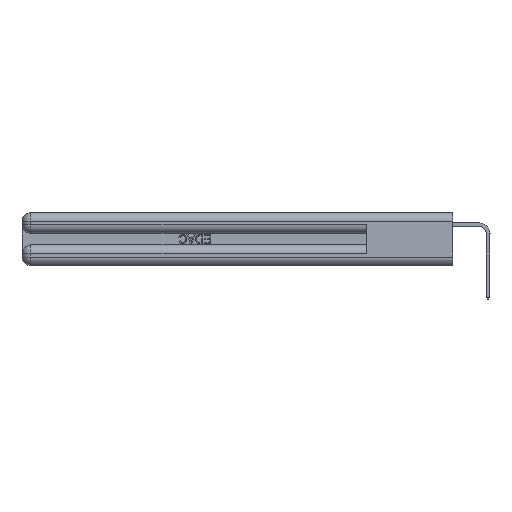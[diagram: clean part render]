
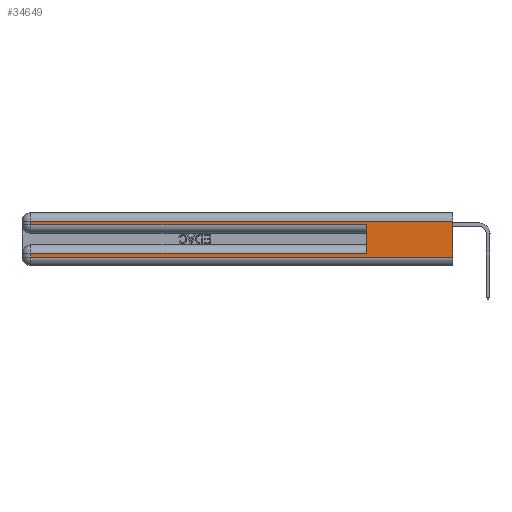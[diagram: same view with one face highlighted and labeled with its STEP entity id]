
A CAD part, left-side view. The second image highlights one B-rep face of the part: STEP entity #34649.
In plain terms, the highlighted planar face has unit normal (-1, 0, 0).
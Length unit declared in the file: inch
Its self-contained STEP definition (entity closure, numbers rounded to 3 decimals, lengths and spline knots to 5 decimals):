
#411 = CARTESIAN_POINT ( 'NONE',  ( 0., 0., 0.06 ) ) ;
#969 = DIRECTION ( 'NONE',  ( 0., 1., 0. ) ) ;
#987 = FACE_OUTER_BOUND ( 'NONE', #24154, .T. ) ;
#1579 = ORIENTED_EDGE ( 'NONE', *, *, #29542, .T. ) ;
#2471 = LINE ( 'NONE', #37907, #32843 ) ;
#2989 = CARTESIAN_POINT ( 'NONE',  ( 0., 0., 0.37 ) ) ;
#3733 = DIRECTION ( 'NONE',  ( 0., 0., -1. ) ) ;
#4904 = CARTESIAN_POINT ( 'NONE',  ( 0., 2.94, 0.06 ) ) ;
#5235 = ORIENTED_EDGE ( 'NONE', *, *, #41045, .F. ) ;
#5409 = VECTOR ( 'NONE', #12151, 39.37008 ) ;
#5661 = CARTESIAN_POINT ( 'NONE',  ( 0., 2.94, 0.085 ) ) ;
#6236 = VERTEX_POINT ( 'NONE', #17973 ) ;
#6950 = DIRECTION ( 'NONE',  ( 0., 0., -1. ) ) ;
#6978 = ORIENTED_EDGE ( 'NONE', *, *, #41016, .T. ) ;
#7427 = VERTEX_POINT ( 'NONE', #27068 ) ;
#8696 = CARTESIAN_POINT ( 'NONE',  ( 0., 0., 0.285 ) ) ;
#11018 = LINE ( 'NONE', #8696, #29640 ) ;
#11496 = CARTESIAN_POINT ( 'NONE',  ( 0., 2.94, 0.37 ) ) ;
#11699 = LINE ( 'NONE', #37723, #31542 ) ;
#12151 = DIRECTION ( 'NONE',  ( 0., -1., 0. ) ) ;
#15657 = CARTESIAN_POINT ( 'NONE',  ( 0., 0., 0.37 ) ) ;
#15744 = VERTEX_POINT ( 'NONE', #34333 ) ;
#15978 = EDGE_CURVE ( 'NONE', #42438, #24179, #35738, .T. ) ;
#16703 = EDGE_CURVE ( 'NONE', #28007, #7427, #41786, .T. ) ;
#17973 = CARTESIAN_POINT ( 'NONE',  ( 0., 0.6, 0.085 ) ) ;
#18443 = ORIENTED_EDGE ( 'NONE', *, *, #16703, .T. ) ;
#18737 = PLANE ( 'NONE',  #23567 ) ;
#23567 = AXIS2_PLACEMENT_3D ( 'NONE', #2989, #30715, #6950 ) ;
#24154 = EDGE_LOOP ( 'NONE', ( #5235, #18443, #36572, #1579, #48325, #49148, #6978, #36566 ) ) ;
#24179 = VERTEX_POINT ( 'NONE', #411 ) ;
#24451 = EDGE_CURVE ( 'NONE', #7427, #15744, #11699, .T. ) ;
#24628 = DIRECTION ( 'NONE',  ( 0., -1., 0. ) ) ;
#25368 = LINE ( 'NONE', #15657, #34647 ) ;
#25998 = DIRECTION ( 'NONE',  ( 0., 1., 0. ) ) ;
#27068 = CARTESIAN_POINT ( 'NONE',  ( 0., 2.94, 0.31 ) ) ;
#27221 = VERTEX_POINT ( 'NONE', #5661 ) ;
#27269 = DIRECTION ( 'NONE',  ( 0., 0., -1. ) ) ;
#27882 = LINE ( 'NONE', #11496, #47515 ) ;
#28007 = VERTEX_POINT ( 'NONE', #50175 ) ;
#29542 = EDGE_CURVE ( 'NONE', #15744, #30012, #11018, .T. ) ;
#29640 = VECTOR ( 'NONE', #24628, 39.37008 ) ;
#30012 = VERTEX_POINT ( 'NONE', #39573 ) ;
#30715 = DIRECTION ( 'NONE',  ( 1., 0., 0. ) ) ;
#31367 = VECTOR ( 'NONE', #969, 39.37008 ) ;
#31542 = VECTOR ( 'NONE', #41663, 39.37008 ) ;
#31800 = LINE ( 'NONE', #45793, #40985 ) ;
#32843 = VECTOR ( 'NONE', #25998, 39.37008 ) ;
#34333 = CARTESIAN_POINT ( 'NONE',  ( 0., 2.94, 0.285 ) ) ;
#34647 = VECTOR ( 'NONE', #3733, 39.37008 ) ;
#34649 = ADVANCED_FACE ( 'NONE', ( #987 ), #18737, .F. ) ;
#35738 = LINE ( 'NONE', #35846, #5409 ) ;
#35846 = CARTESIAN_POINT ( 'NONE',  ( 0., 0., 0.06 ) ) ;
#36225 = EDGE_CURVE ( 'NONE', #6236, #30012, #31800, .T. ) ;
#36566 = ORIENTED_EDGE ( 'NONE', *, *, #15978, .T. ) ;
#36572 = ORIENTED_EDGE ( 'NONE', *, *, #24451, .T. ) ;
#37723 = CARTESIAN_POINT ( 'NONE',  ( 0., 2.94, 0.37 ) ) ;
#37907 = CARTESIAN_POINT ( 'NONE',  ( 0., 0., 0.085 ) ) ;
#38606 = EDGE_CURVE ( 'NONE', #6236, #27221, #2471, .T. ) ;
#39573 = CARTESIAN_POINT ( 'NONE',  ( 0., 0.6, 0.285 ) ) ;
#40985 = VECTOR ( 'NONE', #49725, 39.37008 ) ;
#41016 = EDGE_CURVE ( 'NONE', #27221, #42438, #27882, .T. ) ;
#41045 = EDGE_CURVE ( 'NONE', #28007, #24179, #25368, .T. ) ;
#41663 = DIRECTION ( 'NONE',  ( 0., 0., -1. ) ) ;
#41786 = LINE ( 'NONE', #48209, #31367 ) ;
#42438 = VERTEX_POINT ( 'NONE', #4904 ) ;
#45793 = CARTESIAN_POINT ( 'NONE',  ( 0., 0.6, 0.145 ) ) ;
#47515 = VECTOR ( 'NONE', #27269, 39.37008 ) ;
#48209 = CARTESIAN_POINT ( 'NONE',  ( 0., 0., 0.31 ) ) ;
#48325 = ORIENTED_EDGE ( 'NONE', *, *, #36225, .F. ) ;
#49148 = ORIENTED_EDGE ( 'NONE', *, *, #38606, .T. ) ;
#49725 = DIRECTION ( 'NONE',  ( 0., 0., 1. ) ) ;
#50175 = CARTESIAN_POINT ( 'NONE',  ( 0., 0., 0.31 ) ) ;
